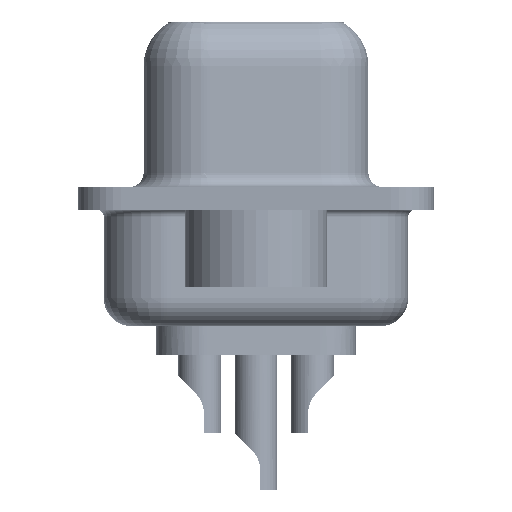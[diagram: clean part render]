
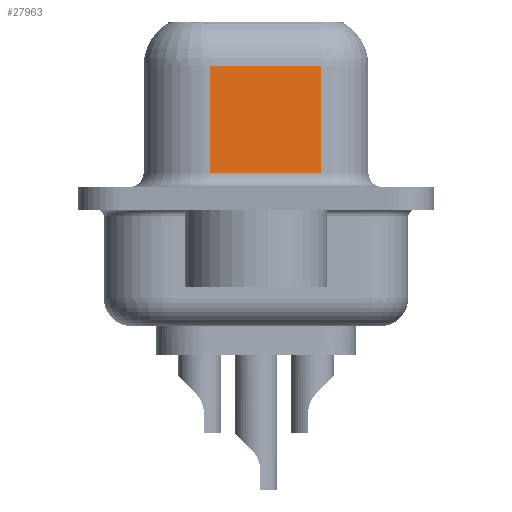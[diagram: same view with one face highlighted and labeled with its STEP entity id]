
A CAD part, left-side view. The second image highlights one B-rep face of the part: STEP entity #27963.
In plain terms, the highlighted planar face has unit normal (-0.985, -0.174, 0).
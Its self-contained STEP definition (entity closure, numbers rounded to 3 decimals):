
#512 = LINE ( 'NONE', #6093, #15491 ) ;
#2172 = EDGE_CURVE ( 'NONE', #3848, #26735, #6774, .T. ) ;
#3380 = CARTESIAN_POINT ( 'NONE',  ( 5.068, -2.297, 4.65 ) ) ;
#3848 = VERTEX_POINT ( 'NONE', #3380 ) ;
#4683 = DIRECTION ( 'NONE',  ( 0.174, -0.985, 0. ) ) ;
#6093 = CARTESIAN_POINT ( 'NONE',  ( 5.068, -2.297, 4.65 ) ) ;
#6774 = LINE ( 'NONE', #26905, #6849 ) ;
#6849 = VECTOR ( 'NONE', #12730, 1000. ) ;
#6902 = DIRECTION ( 'NONE',  ( 0.985, 0.174, 0. ) ) ;
#7268 = CARTESIAN_POINT ( 'NONE',  ( 4.38, 1.603, 6.4 ) ) ;
#7832 = DIRECTION ( 'NONE',  ( 0., 0., -1. ) ) ;
#8105 = AXIS2_PLACEMENT_3D ( 'NONE', #35911, #6902, #21055 ) ;
#9532 = ORIENTED_EDGE ( 'NONE', *, *, #13944, .T. ) ;
#10018 = VERTEX_POINT ( 'NONE', #31025 ) ;
#11605 = VECTOR ( 'NONE', #7832, 1000. ) ;
#12469 = FACE_OUTER_BOUND ( 'NONE', #21168, .T. ) ;
#12730 = DIRECTION ( 'NONE',  ( 0., 0., -1. ) ) ;
#12903 = ORIENTED_EDGE ( 'NONE', *, *, #28394, .T. ) ;
#13944 = EDGE_CURVE ( 'NONE', #10018, #26735, #27693, .T. ) ;
#14762 = VECTOR ( 'NONE', #4683, 1000. ) ;
#14916 = DIRECTION ( 'NONE',  ( -0.174, 0.985, 0. ) ) ;
#15491 = VECTOR ( 'NONE', #14916, 1000. ) ;
#21055 = DIRECTION ( 'NONE',  ( -0.174, 0.985, 0. ) ) ;
#21104 = VERTEX_POINT ( 'NONE', #24511 ) ;
#21168 = EDGE_LOOP ( 'NONE', ( #25162, #12903, #29710, #9532 ) ) ;
#24511 = CARTESIAN_POINT ( 'NONE',  ( 4.38, 1.603, 4.65 ) ) ;
#25162 = ORIENTED_EDGE ( 'NONE', *, *, #2172, .F. ) ;
#25344 = EDGE_CURVE ( 'NONE', #21104, #10018, #31445, .T. ) ;
#26735 = VERTEX_POINT ( 'NONE', #33770 ) ;
#26905 = CARTESIAN_POINT ( 'NONE',  ( 5.068, -2.297, 6.4 ) ) ;
#27693 = LINE ( 'NONE', #31141, #14762 ) ;
#27963 = ADVANCED_FACE ( 'NONE', ( #12469 ), #35721, .F. ) ;
#28394 = EDGE_CURVE ( 'NONE', #3848, #21104, #512, .T. ) ;
#29710 = ORIENTED_EDGE ( 'NONE', *, *, #25344, .T. ) ;
#31025 = CARTESIAN_POINT ( 'NONE',  ( 4.38, 1.603, 0.9 ) ) ;
#31141 = CARTESIAN_POINT ( 'NONE',  ( 5.068, -2.297, 0.9 ) ) ;
#31445 = LINE ( 'NONE', #7268, #11605 ) ;
#33770 = CARTESIAN_POINT ( 'NONE',  ( 5.068, -2.297, 0.9 ) ) ;
#35721 = PLANE ( 'NONE',  #8105 ) ;
#35911 = CARTESIAN_POINT ( 'NONE',  ( 5.068, -2.297, 6.4 ) ) ;
